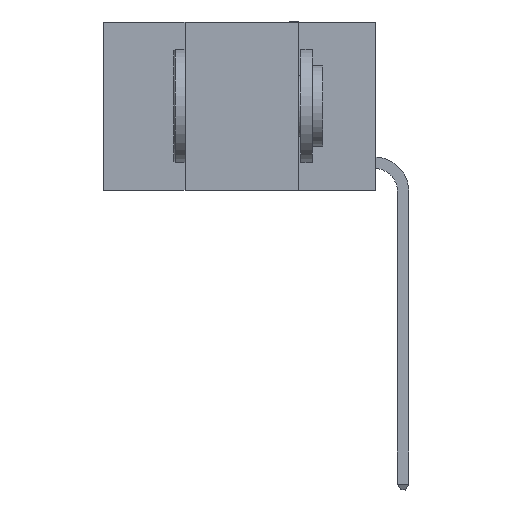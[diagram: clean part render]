
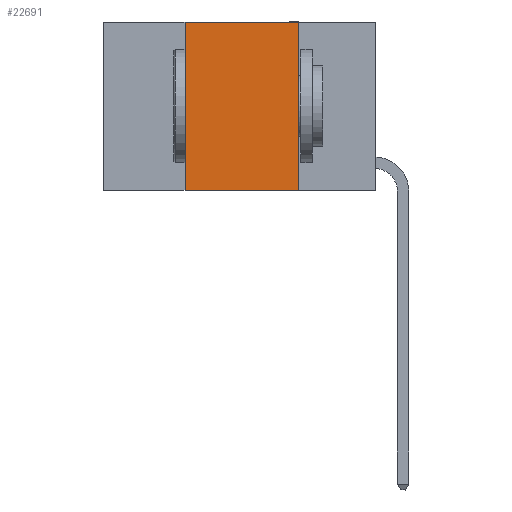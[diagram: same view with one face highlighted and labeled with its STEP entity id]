
A CAD part, left-side view. The second image highlights one B-rep face of the part: STEP entity #22691.
In plain terms, the highlighted planar face has unit normal (-1, 0, 0).
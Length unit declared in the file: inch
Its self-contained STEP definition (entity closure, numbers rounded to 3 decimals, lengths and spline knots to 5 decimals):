
#1087 = CARTESIAN_POINT ( 'NONE',  ( 0., 0.6, 0. ) ) ;
#1610 = CARTESIAN_POINT ( 'NONE',  ( 0., 0.6, -0.37 ) ) ;
#2398 = DIRECTION ( 'NONE',  ( 0., 0., -1. ) ) ;
#2620 = DIRECTION ( 'NONE',  ( 0., 0., -1. ) ) ;
#2945 = AXIS2_PLACEMENT_3D ( 'NONE', #1087, #12714, #2620 ) ;
#3028 = VECTOR ( 'NONE', #7938, 39.37008 ) ;
#4332 = CARTESIAN_POINT ( 'NONE',  ( 0., 0.17, 0. ) ) ;
#6492 = VECTOR ( 'NONE', #12979, 39.37008 ) ;
#6895 = CARTESIAN_POINT ( 'NONE',  ( 0., 0.17, -0.37 ) ) ;
#7938 = DIRECTION ( 'NONE',  ( 0., -1., 0. ) ) ;
#8220 = LINE ( 'NONE', #4332, #8464 ) ;
#8464 = VECTOR ( 'NONE', #2398, 39.37008 ) ;
#8545 = VERTEX_POINT ( 'NONE', #21077 ) ;
#8733 = LINE ( 'NONE', #16301, #22304 ) ;
#9572 = LINE ( 'NONE', #1610, #6492 ) ;
#9832 = LINE ( 'NONE', #17500, #3028 ) ;
#11248 = VERTEX_POINT ( 'NONE', #21355 ) ;
#12714 = DIRECTION ( 'NONE',  ( 1., 0., 0. ) ) ;
#12804 = ORIENTED_EDGE ( 'NONE', *, *, #22825, .F. ) ;
#12954 = ORIENTED_EDGE ( 'NONE', *, *, #17681, .T. ) ;
#12979 = DIRECTION ( 'NONE',  ( 0., -1., 0. ) ) ;
#13668 = VERTEX_POINT ( 'NONE', #6895 ) ;
#15709 = EDGE_CURVE ( 'NONE', #17603, #13668, #8220, .T. ) ;
#16118 = PLANE ( 'NONE',  #2945 ) ;
#16301 = CARTESIAN_POINT ( 'NONE',  ( 0., 0.42, 0. ) ) ;
#17226 = EDGE_LOOP ( 'NONE', ( #23729, #12804, #22186, #12954 ) ) ;
#17500 = CARTESIAN_POINT ( 'NONE',  ( 0., 0.6, 0. ) ) ;
#17603 = VERTEX_POINT ( 'NONE', #24553 ) ;
#17681 = EDGE_CURVE ( 'NONE', #11248, #13668, #9572, .T. ) ;
#18375 = FACE_OUTER_BOUND ( 'NONE', #17226, .T. ) ;
#20336 = DIRECTION ( 'NONE',  ( 0., 0., 1. ) ) ;
#21077 = CARTESIAN_POINT ( 'NONE',  ( 0., 0.42, 0. ) ) ;
#21355 = CARTESIAN_POINT ( 'NONE',  ( 0., 0.42, -0.37 ) ) ;
#21861 = EDGE_CURVE ( 'NONE', #11248, #8545, #8733, .T. ) ;
#22186 = ORIENTED_EDGE ( 'NONE', *, *, #21861, .F. ) ;
#22304 = VECTOR ( 'NONE', #20336, 39.37008 ) ;
#22691 = ADVANCED_FACE ( 'NONE', ( #18375 ), #16118, .F. ) ;
#22825 = EDGE_CURVE ( 'NONE', #8545, #17603, #9832, .T. ) ;
#23729 = ORIENTED_EDGE ( 'NONE', *, *, #15709, .F. ) ;
#24553 = CARTESIAN_POINT ( 'NONE',  ( 0., 0.17, 0. ) ) ;
